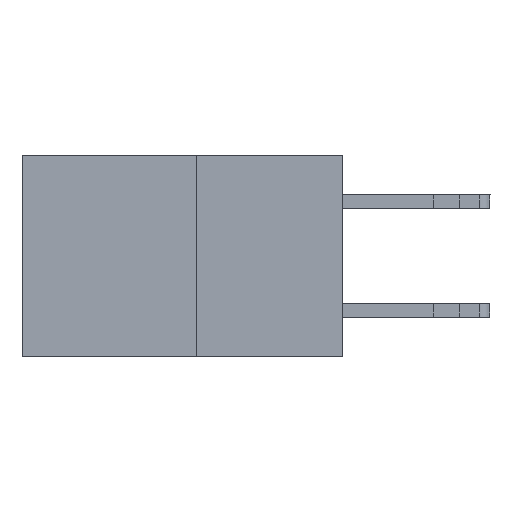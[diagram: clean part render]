
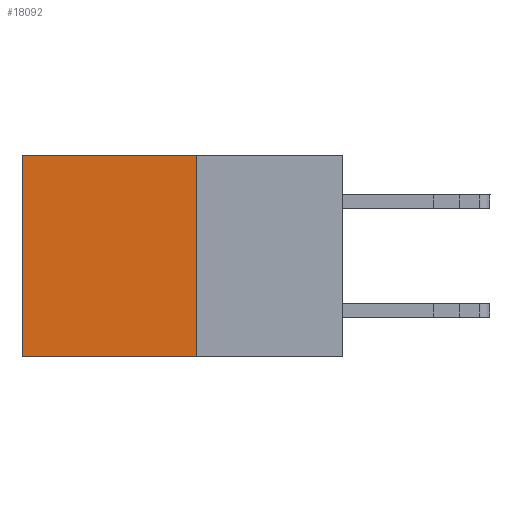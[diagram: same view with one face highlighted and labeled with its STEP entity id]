
A CAD part, left-side view. The second image highlights one B-rep face of the part: STEP entity #18092.
In plain terms, the highlighted planar face has unit normal (-1, 0, 0).
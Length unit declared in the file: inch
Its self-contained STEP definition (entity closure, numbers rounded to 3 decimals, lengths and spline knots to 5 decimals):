
#922 = VECTOR ( 'NONE', #17217, 39.37008 ) ;
#1091 = ORIENTED_EDGE ( 'NONE', *, *, #3387, .F. ) ;
#1782 = ORIENTED_EDGE ( 'NONE', *, *, #12864, .F. ) ;
#2342 = DIRECTION ( 'NONE',  ( 0., 0., -1. ) ) ;
#2709 = VECTOR ( 'NONE', #2852, 39.37008 ) ;
#2852 = DIRECTION ( 'NONE',  ( 0., 1., 0. ) ) ;
#3387 = EDGE_CURVE ( 'NONE', #5606, #8013, #10049, .T. ) ;
#3567 = VECTOR ( 'NONE', #16659, 39.37008 ) ;
#3651 = EDGE_CURVE ( 'NONE', #13623, #14461, #8171, .T. ) ;
#5284 = EDGE_LOOP ( 'NONE', ( #14596, #1091, #1782, #10906 ) ) ;
#5523 = LINE ( 'NONE', #8459, #922 ) ;
#5606 = VERTEX_POINT ( 'NONE', #5781 ) ;
#5607 = VECTOR ( 'NONE', #2342, 39.37008 ) ;
#5781 = CARTESIAN_POINT ( 'NONE',  ( 0.277, 0.27, -0.37 ) ) ;
#5875 = CARTESIAN_POINT ( 'NONE',  ( 0.277, 0.27, -0.37 ) ) ;
#8013 = VERTEX_POINT ( 'NONE', #15631 ) ;
#8171 = LINE ( 'NONE', #11090, #3567 ) ;
#8225 = FACE_OUTER_BOUND ( 'NONE', #5284, .T. ) ;
#8459 = CARTESIAN_POINT ( 'NONE',  ( 0.277, 0.59, -0.37 ) ) ;
#9830 = DIRECTION ( 'NONE',  ( 1., 0., 0. ) ) ;
#10049 = LINE ( 'NONE', #5875, #2709 ) ;
#10906 = ORIENTED_EDGE ( 'NONE', *, *, #3651, .T. ) ;
#10937 = LINE ( 'NONE', #16602, #5607 ) ;
#11090 = CARTESIAN_POINT ( 'NONE',  ( 0.277, 0.27, 0. ) ) ;
#11462 = AXIS2_PLACEMENT_3D ( 'NONE', #12845, #9830, #12760 ) ;
#11533 = EDGE_CURVE ( 'NONE', #14461, #8013, #5523, .T. ) ;
#12760 = DIRECTION ( 'NONE',  ( 0., 0., -1. ) ) ;
#12845 = CARTESIAN_POINT ( 'NONE',  ( 0.277, 0.27, -0.37 ) ) ;
#12864 = EDGE_CURVE ( 'NONE', #13623, #5606, #10937, .T. ) ;
#13623 = VERTEX_POINT ( 'NONE', #17860 ) ;
#14461 = VERTEX_POINT ( 'NONE', #17911 ) ;
#14596 = ORIENTED_EDGE ( 'NONE', *, *, #11533, .T. ) ;
#15631 = CARTESIAN_POINT ( 'NONE',  ( 0.277, 0.59, -0.37 ) ) ;
#16602 = CARTESIAN_POINT ( 'NONE',  ( 0.277, 0.27, -0.37 ) ) ;
#16659 = DIRECTION ( 'NONE',  ( 0., 1., 0. ) ) ;
#16992 = PLANE ( 'NONE',  #11462 ) ;
#17217 = DIRECTION ( 'NONE',  ( 0., 0., -1. ) ) ;
#17860 = CARTESIAN_POINT ( 'NONE',  ( 0.277, 0.27, 0. ) ) ;
#17911 = CARTESIAN_POINT ( 'NONE',  ( 0.277, 0.59, 0. ) ) ;
#18092 = ADVANCED_FACE ( 'NONE', ( #8225 ), #16992, .F. ) ;
